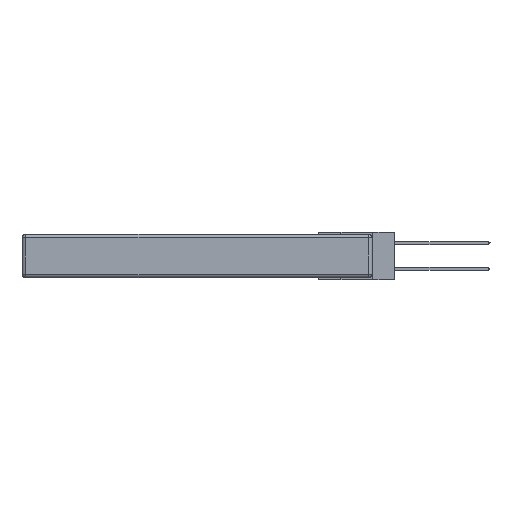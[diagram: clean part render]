
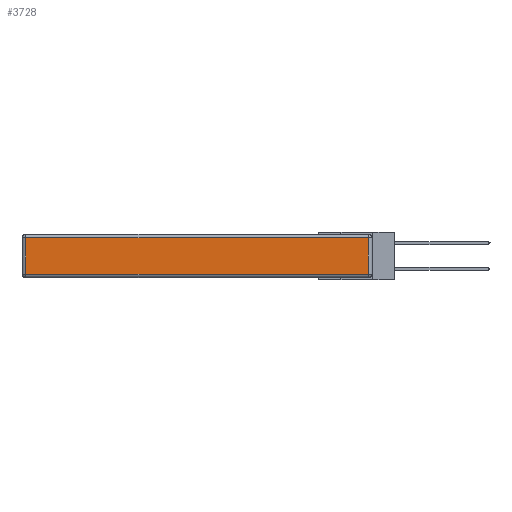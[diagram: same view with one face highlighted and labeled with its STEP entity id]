
A CAD part, left-side view. The second image highlights one B-rep face of the part: STEP entity #3728.
In plain terms, the highlighted planar face has unit normal (-1, 0, 0).
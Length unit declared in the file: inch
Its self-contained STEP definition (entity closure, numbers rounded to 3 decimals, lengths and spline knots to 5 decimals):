
#458 = EDGE_CURVE ( 'NONE', #27312, #1557, #22589, .T. ) ;
#1533 = PLANE ( 'NONE',  #6585 ) ;
#1557 = VERTEX_POINT ( 'NONE', #8578 ) ;
#3728 = ADVANCED_FACE ( 'NONE', ( #11359 ), #1533, .T. ) ;
#3946 = DIRECTION ( 'NONE',  ( 0., 0., 1. ) ) ;
#4165 = DIRECTION ( 'NONE',  ( 0., 0., -1. ) ) ;
#6585 = AXIS2_PLACEMENT_3D ( 'NONE', #19546, #28494, #3946 ) ;
#6643 = DIRECTION ( 'NONE',  ( 0., 0., 1. ) ) ;
#7395 = CARTESIAN_POINT ( 'NONE',  ( 0., 2.75, -0.03 ) ) ;
#7710 = ORIENTED_EDGE ( 'NONE', *, *, #19866, .T. ) ;
#8578 = CARTESIAN_POINT ( 'NONE',  ( 0., 0.03, -0.03 ) ) ;
#8620 = CARTESIAN_POINT ( 'NONE',  ( 0., 2.72, -0.313 ) ) ;
#8933 = VECTOR ( 'NONE', #6643, 39.37008 ) ;
#9908 = LINE ( 'NONE', #10572, #20769 ) ;
#10572 = CARTESIAN_POINT ( 'NONE',  ( 0., 2.72, -0.343 ) ) ;
#10589 = CARTESIAN_POINT ( 'NONE',  ( 0., 0., -0.313 ) ) ;
#11359 = FACE_OUTER_BOUND ( 'NONE', #26780, .T. ) ;
#12400 = VECTOR ( 'NONE', #18889, 39.37008 ) ;
#12828 = LINE ( 'NONE', #10589, #17747 ) ;
#14470 = ORIENTED_EDGE ( 'NONE', *, *, #14989, .T. ) ;
#14573 = ORIENTED_EDGE ( 'NONE', *, *, #22494, .T. ) ;
#14770 = VERTEX_POINT ( 'NONE', #8620 ) ;
#14989 = EDGE_CURVE ( 'NONE', #1557, #24467, #24298, .T. ) ;
#15632 = CARTESIAN_POINT ( 'NONE',  ( 0., 0.03, -0.343 ) ) ;
#17035 = CARTESIAN_POINT ( 'NONE',  ( 0., 2.72, -0.03 ) ) ;
#17747 = VECTOR ( 'NONE', #28553, 39.37008 ) ;
#18889 = DIRECTION ( 'NONE',  ( 0., 1., 0. ) ) ;
#19546 = CARTESIAN_POINT ( 'NONE',  ( 0., 0., -0.343 ) ) ;
#19866 = EDGE_CURVE ( 'NONE', #14770, #27312, #12828, .T. ) ;
#20769 = VECTOR ( 'NONE', #4165, 39.37008 ) ;
#22494 = EDGE_CURVE ( 'NONE', #24467, #14770, #9908, .T. ) ;
#22589 = LINE ( 'NONE', #15632, #8933 ) ;
#24298 = LINE ( 'NONE', #7395, #12400 ) ;
#24416 = ORIENTED_EDGE ( 'NONE', *, *, #458, .T. ) ;
#24467 = VERTEX_POINT ( 'NONE', #17035 ) ;
#25664 = CARTESIAN_POINT ( 'NONE',  ( 0., 0.03, -0.313 ) ) ;
#26780 = EDGE_LOOP ( 'NONE', ( #7710, #24416, #14470, #14573 ) ) ;
#27312 = VERTEX_POINT ( 'NONE', #25664 ) ;
#28494 = DIRECTION ( 'NONE',  ( -1., 0., 0. ) ) ;
#28553 = DIRECTION ( 'NONE',  ( 0., -1., 0. ) ) ;
